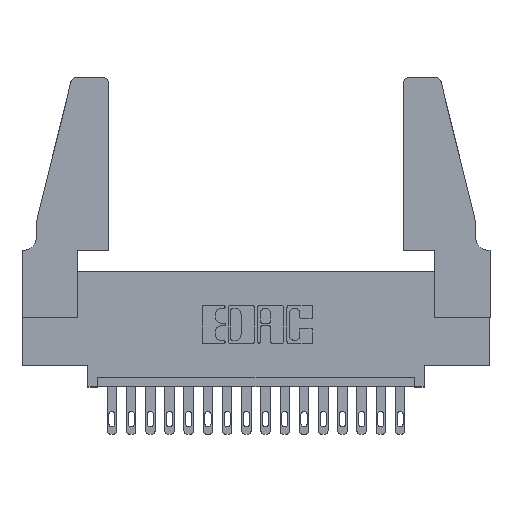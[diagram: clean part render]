
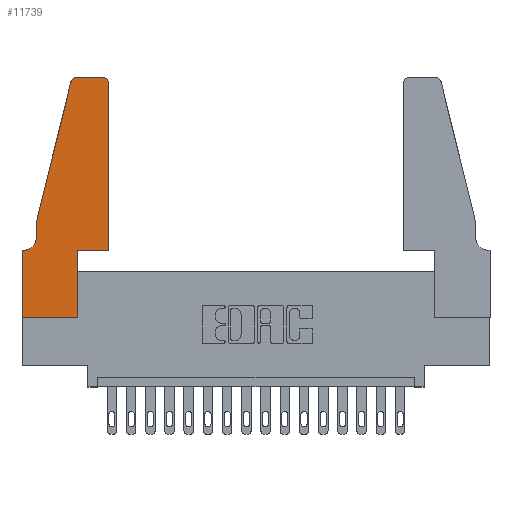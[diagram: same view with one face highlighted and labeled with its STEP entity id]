
A CAD part, top view. The second image highlights one B-rep face of the part: STEP entity #11739.
In plain terms, the highlighted planar face has unit normal (0, 0, 1).
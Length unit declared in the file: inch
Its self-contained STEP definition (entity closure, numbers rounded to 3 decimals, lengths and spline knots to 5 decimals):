
#288 = CARTESIAN_POINT ( 'NONE',  ( 0.0755, 0.5, 0.37 ) ) ;
#324 = CARTESIAN_POINT ( 'NONE',  ( 0.284, 1.22, 0.37 ) ) ;
#456 = VERTEX_POINT ( 'NONE', #4612 ) ;
#479 = ORIENTED_EDGE ( 'NONE', *, *, #15868, .T. ) ;
#538 = CARTESIAN_POINT ( 'NONE',  ( 0.0755, 0.5, 0.37 ) ) ;
#1114 = CARTESIAN_POINT ( 'NONE',  ( 0.0755, 0.42, 0.37 ) ) ;
#1209 = ORIENTED_EDGE ( 'NONE', *, *, #13502, .T. ) ;
#1295 = VERTEX_POINT ( 'NONE', #13942 ) ;
#1482 = DIRECTION ( 'NONE',  ( 0., 0., 1. ) ) ;
#1666 = CARTESIAN_POINT ( 'NONE',  ( 0.2605, 1.25, 0.37 ) ) ;
#1905 = AXIS2_PLACEMENT_3D ( 'NONE', #14844, #6598, #17542 ) ;
#2195 = DIRECTION ( 'NONE',  ( -1., 0., 0. ) ) ;
#2465 = FACE_OUTER_BOUND ( 'NONE', #4455, .T. ) ;
#2707 = CARTESIAN_POINT ( 'NONE',  ( 0.2865, 0., 0.37 ) ) ;
#2891 = EDGE_CURVE ( 'NONE', #7776, #4160, #15190, .T. ) ;
#3010 = DIRECTION ( 'NONE',  ( 0., 1., 0. ) ) ;
#3083 = AXIS2_PLACEMENT_3D ( 'NONE', #324, #4526, #9858 ) ;
#3229 = DIRECTION ( 'NONE',  ( -1., 0., 0. ) ) ;
#3554 = CIRCLE ( 'NONE', #1905, 0.07 ) ;
#3602 = CARTESIAN_POINT ( 'NONE',  ( 0., 0., 0.37 ) ) ;
#3657 = LINE ( 'NONE', #3602, #9215 ) ;
#3682 = VERTEX_POINT ( 'NONE', #14316 ) ;
#3711 = VECTOR ( 'NONE', #9134, 39.37008 ) ;
#3938 = EDGE_CURVE ( 'NONE', #7315, #4543, #6733, .T. ) ;
#4160 = VERTEX_POINT ( 'NONE', #11464 ) ;
#4455 = EDGE_LOOP ( 'NONE', ( #11256, #11563, #6462, #11047, #4616, #4798, #479, #14228, #16870, #6871, #1209, #9697 ) ) ;
#4526 = DIRECTION ( 'NONE',  ( 0., 0., 1. ) ) ;
#4543 = VERTEX_POINT ( 'NONE', #2707 ) ;
#4612 = CARTESIAN_POINT ( 'NONE',  ( 0., 0.35, 0.37 ) ) ;
#4616 = ORIENTED_EDGE ( 'NONE', *, *, #11376, .T. ) ;
#4655 = CARTESIAN_POINT ( 'NONE',  ( 0.0755, 0.35, 0.37 ) ) ;
#4694 = CARTESIAN_POINT ( 'NONE',  ( 0., 0.35, 0.37 ) ) ;
#4755 = DIRECTION ( 'NONE',  ( 1., 0., 0. ) ) ;
#4798 = ORIENTED_EDGE ( 'NONE', *, *, #9248, .T. ) ;
#4847 = CARTESIAN_POINT ( 'NONE',  ( 0.284, 1.25, 0.37 ) ) ;
#4862 = CARTESIAN_POINT ( 'NONE',  ( 0., 0., 0.37 ) ) ;
#4908 = CIRCLE ( 'NONE', #9397, 0.03 ) ;
#5054 = VECTOR ( 'NONE', #5860, 39.37008 ) ;
#5423 = VECTOR ( 'NONE', #10444, 39.37008 ) ;
#5639 = CARTESIAN_POINT ( 'NONE',  ( 0.2865, 0.35, 0.37 ) ) ;
#5860 = DIRECTION ( 'NONE',  ( -0.239, -0.971, 0. ) ) ;
#5898 = CARTESIAN_POINT ( 'NONE',  ( 0.4505, 0.35, 0.37 ) ) ;
#6225 = LINE ( 'NONE', #5639, #6662 ) ;
#6444 = CARTESIAN_POINT ( 'NONE',  ( 0.25487, 1.22718, 0.37 ) ) ;
#6462 = ORIENTED_EDGE ( 'NONE', *, *, #2891, .T. ) ;
#6598 = DIRECTION ( 'NONE',  ( 0., 0., -1. ) ) ;
#6662 = VECTOR ( 'NONE', #3010, 39.37008 ) ;
#6715 = VERTEX_POINT ( 'NONE', #11675 ) ;
#6733 = LINE ( 'NONE', #4862, #5423 ) ;
#6871 = ORIENTED_EDGE ( 'NONE', *, *, #11277, .T. ) ;
#7126 = LINE ( 'NONE', #10746, #3711 ) ;
#7277 = LINE ( 'NONE', #538, #16316 ) ;
#7315 = VERTEX_POINT ( 'NONE', #14953 ) ;
#7776 = VERTEX_POINT ( 'NONE', #6444 ) ;
#8060 = VERTEX_POINT ( 'NONE', #4847 ) ;
#8476 = LINE ( 'NONE', #10873, #17313 ) ;
#9132 = EDGE_CURVE ( 'NONE', #4160, #17182, #7277, .T. ) ;
#9134 = DIRECTION ( 'NONE',  ( 0., 1., 0. ) ) ;
#9215 = VECTOR ( 'NONE', #13132, 39.37008 ) ;
#9248 = EDGE_CURVE ( 'NONE', #1295, #456, #12620, .T. ) ;
#9397 = AXIS2_PLACEMENT_3D ( 'NONE', #9686, #1482, #11054 ) ;
#9686 = CARTESIAN_POINT ( 'NONE',  ( 0.4205, 1.22, 0.37 ) ) ;
#9697 = ORIENTED_EDGE ( 'NONE', *, *, #16695, .T. ) ;
#9858 = DIRECTION ( 'NONE',  ( 1., 0., 0. ) ) ;
#9974 = VECTOR ( 'NONE', #3229, 39.37008 ) ;
#10381 = VERTEX_POINT ( 'NONE', #5898 ) ;
#10412 = AXIS2_PLACEMENT_3D ( 'NONE', #4694, #12850, #4755 ) ;
#10444 = DIRECTION ( 'NONE',  ( 1., 0., 0. ) ) ;
#10698 = VECTOR ( 'NONE', #2195, 39.37008 ) ;
#10746 = CARTESIAN_POINT ( 'NONE',  ( 0.4505, 0.35, 0.37 ) ) ;
#10873 = CARTESIAN_POINT ( 'NONE',  ( 0.4505, 0.35, 0.37 ) ) ;
#11047 = ORIENTED_EDGE ( 'NONE', *, *, #9132, .T. ) ;
#11054 = DIRECTION ( 'NONE',  ( 1., 0., 0. ) ) ;
#11256 = ORIENTED_EDGE ( 'NONE', *, *, #11482, .T. ) ;
#11277 = EDGE_CURVE ( 'NONE', #6715, #10381, #8476, .T. ) ;
#11376 = EDGE_CURVE ( 'NONE', #17182, #1295, #3554, .T. ) ;
#11464 = CARTESIAN_POINT ( 'NONE',  ( 0.0755, 0.5, 0.37 ) ) ;
#11482 = EDGE_CURVE ( 'NONE', #3682, #8060, #13620, .T. ) ;
#11563 = ORIENTED_EDGE ( 'NONE', *, *, #15080, .T. ) ;
#11675 = CARTESIAN_POINT ( 'NONE',  ( 0.2865, 0.35, 0.37 ) ) ;
#11739 = ADVANCED_FACE ( 'NONE', ( #2465 ), #14303, .T. ) ;
#12620 = LINE ( 'NONE', #4655, #10698 ) ;
#12850 = DIRECTION ( 'NONE',  ( 0., 0., 1. ) ) ;
#13132 = DIRECTION ( 'NONE',  ( 0., -1., 0. ) ) ;
#13502 = EDGE_CURVE ( 'NONE', #10381, #16172, #7126, .T. ) ;
#13620 = LINE ( 'NONE', #1666, #9974 ) ;
#13942 = CARTESIAN_POINT ( 'NONE',  ( 0.0055, 0.35, 0.37 ) ) ;
#14228 = ORIENTED_EDGE ( 'NONE', *, *, #3938, .T. ) ;
#14303 = PLANE ( 'NONE',  #10412 ) ;
#14316 = CARTESIAN_POINT ( 'NONE',  ( 0.4205, 1.25, 0.37 ) ) ;
#14844 = CARTESIAN_POINT ( 'NONE',  ( 0.0055, 0.42, 0.37 ) ) ;
#14884 = CIRCLE ( 'NONE', #3083, 0.03 ) ;
#14953 = CARTESIAN_POINT ( 'NONE',  ( 0., 0., 0.37 ) ) ;
#15080 = EDGE_CURVE ( 'NONE', #8060, #7776, #14884, .T. ) ;
#15190 = LINE ( 'NONE', #288, #5054 ) ;
#15602 = EDGE_CURVE ( 'NONE', #4543, #6715, #6225, .T. ) ;
#15868 = EDGE_CURVE ( 'NONE', #456, #7315, #3657, .T. ) ;
#16172 = VERTEX_POINT ( 'NONE', #17767 ) ;
#16316 = VECTOR ( 'NONE', #16935, 39.37008 ) ;
#16695 = EDGE_CURVE ( 'NONE', #16172, #3682, #4908, .T. ) ;
#16870 = ORIENTED_EDGE ( 'NONE', *, *, #15602, .T. ) ;
#16935 = DIRECTION ( 'NONE',  ( 0., -1., 0. ) ) ;
#17182 = VERTEX_POINT ( 'NONE', #1114 ) ;
#17313 = VECTOR ( 'NONE', #17615, 39.37008 ) ;
#17542 = DIRECTION ( 'NONE',  ( -1., 0., 0. ) ) ;
#17615 = DIRECTION ( 'NONE',  ( 1., 0., 0. ) ) ;
#17767 = CARTESIAN_POINT ( 'NONE',  ( 0.4505, 1.22, 0.37 ) ) ;
